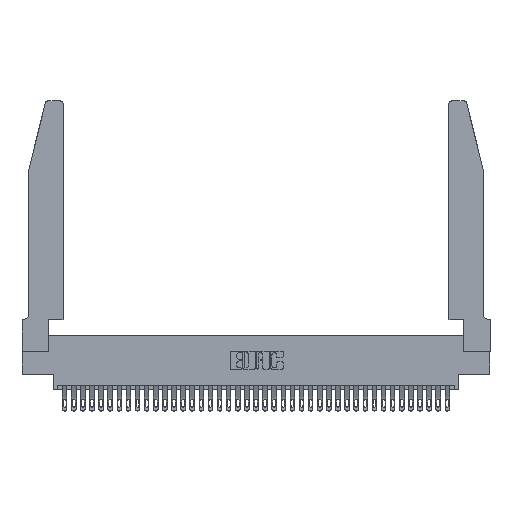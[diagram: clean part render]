
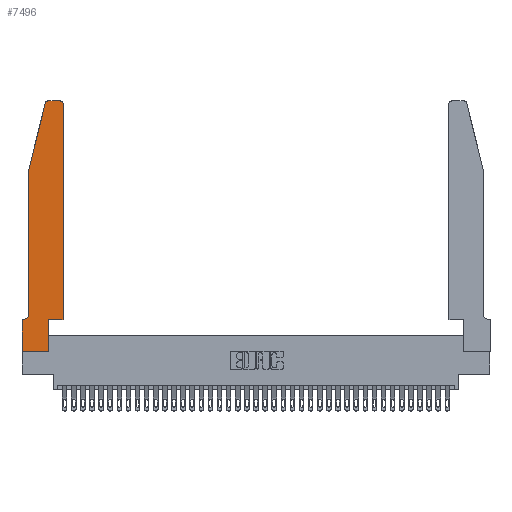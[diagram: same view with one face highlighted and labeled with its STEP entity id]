
A CAD part, top view. The second image highlights one B-rep face of the part: STEP entity #7496.
In plain terms, the highlighted planar face has unit normal (0, 0, 1).
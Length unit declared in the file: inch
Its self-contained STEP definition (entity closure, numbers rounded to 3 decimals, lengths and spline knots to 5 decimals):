
#1130 = CARTESIAN_POINT ( 'NONE',  ( 0.4205, 2.72, 0.37 ) ) ;
#1139 = EDGE_CURVE ( 'NONE', #29701, #9617, #2761, .T. ) ;
#1493 = CIRCLE ( 'NONE', #23879, 0.07 ) ;
#1559 = CARTESIAN_POINT ( 'NONE',  ( 0.2605, 2.75, 0.37 ) ) ;
#1691 = ORIENTED_EDGE ( 'NONE', *, *, #11585, .T. ) ;
#1928 = CARTESIAN_POINT ( 'NONE',  ( 0.4505, 0.35, 0.37 ) ) ;
#2051 = VERTEX_POINT ( 'NONE', #4966 ) ;
#2761 = LINE ( 'NONE', #28390, #29507 ) ;
#2983 = VERTEX_POINT ( 'NONE', #25828 ) ;
#3080 = ORIENTED_EDGE ( 'NONE', *, *, #30414, .T. ) ;
#3085 = CARTESIAN_POINT ( 'NONE',  ( 0., 0., 0.37 ) ) ;
#4804 = VERTEX_POINT ( 'NONE', #11258 ) ;
#4851 = DIRECTION ( 'NONE',  ( -1., 0., 0. ) ) ;
#4966 = CARTESIAN_POINT ( 'NONE',  ( 0.0755, 0.42, 0.37 ) ) ;
#4979 = DIRECTION ( 'NONE',  ( 0., 0., 1. ) ) ;
#5018 = ORIENTED_EDGE ( 'NONE', *, *, #19555, .T. ) ;
#5423 = CARTESIAN_POINT ( 'NONE',  ( 0.2865, 0., 0.37 ) ) ;
#5644 = CARTESIAN_POINT ( 'NONE',  ( 0.2865, 0.35, 0.37 ) ) ;
#5694 = VERTEX_POINT ( 'NONE', #29145 ) ;
#5740 = VECTOR ( 'NONE', #28515, 39.37008 ) ;
#5793 = ORIENTED_EDGE ( 'NONE', *, *, #29946, .T. ) ;
#6498 = CARTESIAN_POINT ( 'NONE',  ( 0.4505, 0.35, 0.37 ) ) ;
#6797 = VERTEX_POINT ( 'NONE', #14992 ) ;
#7195 = DIRECTION ( 'NONE',  ( 1., 0., 0. ) ) ;
#7496 = ADVANCED_FACE ( 'NONE', ( #35164 ), #14118, .T. ) ;
#8022 = CARTESIAN_POINT ( 'NONE',  ( 0.25487, 2.72718, 0.37 ) ) ;
#8469 = CIRCLE ( 'NONE', #35030, 0.03 ) ;
#9519 = LINE ( 'NONE', #12710, #9978 ) ;
#9617 = VERTEX_POINT ( 'NONE', #20187 ) ;
#9978 = VECTOR ( 'NONE', #33721, 39.37008 ) ;
#11258 = CARTESIAN_POINT ( 'NONE',  ( 0.4205, 2.75, 0.37 ) ) ;
#11401 = CARTESIAN_POINT ( 'NONE',  ( 0., 0.35, 0.37 ) ) ;
#11585 = EDGE_CURVE ( 'NONE', #12082, #4804, #8469, .T. ) ;
#11723 = ORIENTED_EDGE ( 'NONE', *, *, #19780, .T. ) ;
#12082 = VERTEX_POINT ( 'NONE', #19535 ) ;
#12710 = CARTESIAN_POINT ( 'NONE',  ( 0.0755, 0.35, 0.37 ) ) ;
#13207 = ORIENTED_EDGE ( 'NONE', *, *, #15812, .T. ) ;
#13449 = VERTEX_POINT ( 'NONE', #27867 ) ;
#13739 = VERTEX_POINT ( 'NONE', #18968 ) ;
#14118 = PLANE ( 'NONE',  #32894 ) ;
#14783 = CARTESIAN_POINT ( 'NONE',  ( 0.284, 2.72, 0.37 ) ) ;
#14992 = CARTESIAN_POINT ( 'NONE',  ( 0.0055, 0.35, 0.37 ) ) ;
#15041 = DIRECTION ( 'NONE',  ( 0., 0., 1. ) ) ;
#15143 = LINE ( 'NONE', #1559, #26436 ) ;
#15812 = EDGE_CURVE ( 'NONE', #13449, #20833, #25908, .T. ) ;
#16141 = DIRECTION ( 'NONE',  ( -1., 0., 0. ) ) ;
#16727 = DIRECTION ( 'NONE',  ( 1., 0., 0. ) ) ;
#16771 = VECTOR ( 'NONE', #16727, 39.37008 ) ;
#16863 = EDGE_CURVE ( 'NONE', #4804, #13739, #15143, .T. ) ;
#16908 = CARTESIAN_POINT ( 'NONE',  ( 0.4505, 0.35, 0.37 ) ) ;
#18014 = CARTESIAN_POINT ( 'NONE',  ( 0.0055, 0.42, 0.37 ) ) ;
#18909 = DIRECTION ( 'NONE',  ( -0.239, -0.971, 0. ) ) ;
#18968 = CARTESIAN_POINT ( 'NONE',  ( 0.284, 2.75, 0.37 ) ) ;
#19104 = EDGE_CURVE ( 'NONE', #5694, #2983, #22444, .T. ) ;
#19535 = CARTESIAN_POINT ( 'NONE',  ( 0.4505, 2.72, 0.37 ) ) ;
#19555 = EDGE_CURVE ( 'NONE', #2983, #35946, #20050, .T. ) ;
#19780 = EDGE_CURVE ( 'NONE', #35946, #13449, #31390, .T. ) ;
#19870 = EDGE_CURVE ( 'NONE', #13739, #29701, #27647, .T. ) ;
#20050 = LINE ( 'NONE', #37862, #16771 ) ;
#20118 = DIRECTION ( 'NONE',  ( 0., 1., 0. ) ) ;
#20131 = ORIENTED_EDGE ( 'NONE', *, *, #19104, .T. ) ;
#20187 = CARTESIAN_POINT ( 'NONE',  ( 0.0755, 2., 0.37 ) ) ;
#20210 = VECTOR ( 'NONE', #26400, 39.37008 ) ;
#20833 = VERTEX_POINT ( 'NONE', #16908 ) ;
#21567 = ORIENTED_EDGE ( 'NONE', *, *, #34169, .T. ) ;
#22429 = ORIENTED_EDGE ( 'NONE', *, *, #1139, .T. ) ;
#22444 = LINE ( 'NONE', #3085, #37035 ) ;
#23879 = AXIS2_PLACEMENT_3D ( 'NONE', #18014, #27003, #16141 ) ;
#25044 = ORIENTED_EDGE ( 'NONE', *, *, #31480, .T. ) ;
#25162 = DIRECTION ( 'NONE',  ( 0., 0., 1. ) ) ;
#25641 = VECTOR ( 'NONE', #20118, 39.37008 ) ;
#25828 = CARTESIAN_POINT ( 'NONE',  ( 0., 0., 0.37 ) ) ;
#25908 = LINE ( 'NONE', #6498, #5740 ) ;
#26366 = LINE ( 'NONE', #38567, #20210 ) ;
#26400 = DIRECTION ( 'NONE',  ( 0., -1., 0. ) ) ;
#26436 = VECTOR ( 'NONE', #4851, 39.37008 ) ;
#27003 = DIRECTION ( 'NONE',  ( 0., 0., -1. ) ) ;
#27647 = CIRCLE ( 'NONE', #37919, 0.03 ) ;
#27867 = CARTESIAN_POINT ( 'NONE',  ( 0.2865, 0.35, 0.37 ) ) ;
#28390 = CARTESIAN_POINT ( 'NONE',  ( 0.0755, 2., 0.37 ) ) ;
#28485 = LINE ( 'NONE', #1928, #25641 ) ;
#28515 = DIRECTION ( 'NONE',  ( 1., 0., 0. ) ) ;
#28566 = ORIENTED_EDGE ( 'NONE', *, *, #19870, .T. ) ;
#29145 = CARTESIAN_POINT ( 'NONE',  ( 0., 0.35, 0.37 ) ) ;
#29507 = VECTOR ( 'NONE', #18909, 39.37008 ) ;
#29701 = VERTEX_POINT ( 'NONE', #8022 ) ;
#29946 = EDGE_CURVE ( 'NONE', #6797, #5694, #9519, .T. ) ;
#30414 = EDGE_CURVE ( 'NONE', #2051, #6797, #1493, .T. ) ;
#30435 = VECTOR ( 'NONE', #35277, 39.37008 ) ;
#31390 = LINE ( 'NONE', #5644, #30435 ) ;
#31480 = EDGE_CURVE ( 'NONE', #9617, #2051, #26366, .T. ) ;
#32865 = DIRECTION ( 'NONE',  ( 0., -1., 0. ) ) ;
#32894 = AXIS2_PLACEMENT_3D ( 'NONE', #11401, #4979, #34898 ) ;
#32905 = ORIENTED_EDGE ( 'NONE', *, *, #16863, .T. ) ;
#33721 = DIRECTION ( 'NONE',  ( -1., 0., 0. ) ) ;
#34169 = EDGE_CURVE ( 'NONE', #20833, #12082, #28485, .T. ) ;
#34898 = DIRECTION ( 'NONE',  ( 1., 0., 0. ) ) ;
#35030 = AXIS2_PLACEMENT_3D ( 'NONE', #1130, #25162, #7195 ) ;
#35164 = FACE_OUTER_BOUND ( 'NONE', #37100, .T. ) ;
#35277 = DIRECTION ( 'NONE',  ( 0., 1., 0. ) ) ;
#35946 = VERTEX_POINT ( 'NONE', #5423 ) ;
#36056 = DIRECTION ( 'NONE',  ( 1., 0., 0. ) ) ;
#37035 = VECTOR ( 'NONE', #32865, 39.37008 ) ;
#37100 = EDGE_LOOP ( 'NONE', ( #32905, #28566, #22429, #25044, #3080, #5793, #20131, #5018, #11723, #13207, #21567, #1691 ) ) ;
#37862 = CARTESIAN_POINT ( 'NONE',  ( 0., 0., 0.37 ) ) ;
#37919 = AXIS2_PLACEMENT_3D ( 'NONE', #14783, #15041, #36056 ) ;
#38567 = CARTESIAN_POINT ( 'NONE',  ( 0.0755, 2., 0.37 ) ) ;
